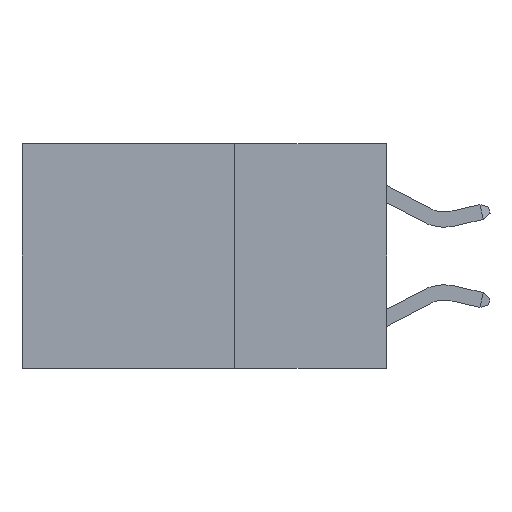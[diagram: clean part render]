
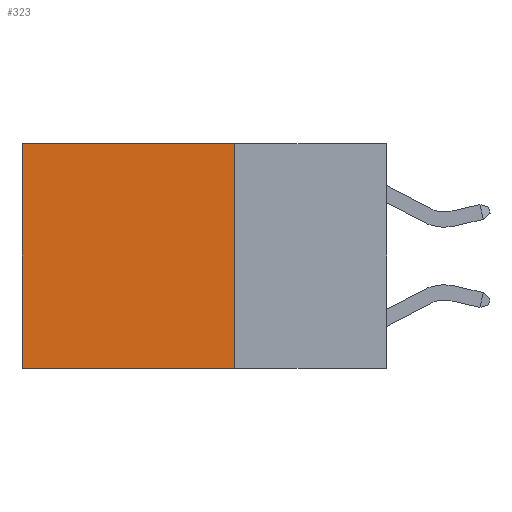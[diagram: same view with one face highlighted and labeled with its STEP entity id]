
A CAD part, left-side view. The second image highlights one B-rep face of the part: STEP entity #323.
In plain terms, the highlighted planar face has unit normal (-1, 0, 0).
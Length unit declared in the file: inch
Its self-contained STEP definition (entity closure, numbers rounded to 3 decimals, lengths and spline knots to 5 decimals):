
#47 = EDGE_CURVE ( 'NONE', #4395, #8776, #652, .T. ) ;
#245 = DIRECTION ( 'NONE',  ( 0., 1., 0. ) ) ;
#276 = VECTOR ( 'NONE', #245, 39.37008 ) ;
#323 = ADVANCED_FACE ( 'NONE', ( #2321 ), #8153, .F. ) ;
#652 = LINE ( 'NONE', #1391, #6294 ) ;
#1089 = VERTEX_POINT ( 'NONE', #1282 ) ;
#1282 = CARTESIAN_POINT ( 'NONE',  ( 0.2625, 0.6, 0. ) ) ;
#1391 = CARTESIAN_POINT ( 'NONE',  ( 0.2625, 0.25, 0. ) ) ;
#1537 = ORIENTED_EDGE ( 'NONE', *, *, #47, .F. ) ;
#1599 = CARTESIAN_POINT ( 'NONE',  ( 0.2625, 0.25, 0. ) ) ;
#1648 = EDGE_CURVE ( 'NONE', #8776, #8783, #3043, .T. ) ;
#1809 = CARTESIAN_POINT ( 'NONE',  ( 0.2625, 0.25, 0. ) ) ;
#2150 = LINE ( 'NONE', #5111, #7468 ) ;
#2187 = ORIENTED_EDGE ( 'NONE', *, *, #1648, .F. ) ;
#2321 = FACE_OUTER_BOUND ( 'NONE', #5531, .T. ) ;
#2572 = DIRECTION ( 'NONE',  ( 0., 0., -1. ) ) ;
#2839 = EDGE_CURVE ( 'NONE', #1089, #8783, #8261, .T. ) ;
#3043 = LINE ( 'NONE', #3908, #276 ) ;
#3132 = DIRECTION ( 'NONE',  ( 0., 1., 0. ) ) ;
#3908 = CARTESIAN_POINT ( 'NONE',  ( 0.2625, 0.25, -0.37 ) ) ;
#4324 = DIRECTION ( 'NONE',  ( 0., 0., -1. ) ) ;
#4357 = CARTESIAN_POINT ( 'NONE',  ( 0.2625, 0.25, -0.37 ) ) ;
#4395 = VERTEX_POINT ( 'NONE', #1809 ) ;
#5111 = CARTESIAN_POINT ( 'NONE',  ( 0.2625, 0.25, 0. ) ) ;
#5531 = EDGE_LOOP ( 'NONE', ( #7903, #2187, #1537, #7173 ) ) ;
#6037 = EDGE_CURVE ( 'NONE', #4395, #1089, #2150, .T. ) ;
#6179 = CARTESIAN_POINT ( 'NONE',  ( 0.2625, 0.6, 0. ) ) ;
#6294 = VECTOR ( 'NONE', #4324, 39.37008 ) ;
#6796 = DIRECTION ( 'NONE',  ( 1., 0., 0. ) ) ;
#6907 = AXIS2_PLACEMENT_3D ( 'NONE', #1599, #6796, #8248 ) ;
#7173 = ORIENTED_EDGE ( 'NONE', *, *, #6037, .T. ) ;
#7468 = VECTOR ( 'NONE', #3132, 39.37008 ) ;
#7878 = CARTESIAN_POINT ( 'NONE',  ( 0.2625, 0.6, -0.37 ) ) ;
#7903 = ORIENTED_EDGE ( 'NONE', *, *, #2839, .T. ) ;
#8153 = PLANE ( 'NONE',  #6907 ) ;
#8248 = DIRECTION ( 'NONE',  ( 0., 0., -1. ) ) ;
#8261 = LINE ( 'NONE', #6179, #8292 ) ;
#8292 = VECTOR ( 'NONE', #2572, 39.37008 ) ;
#8776 = VERTEX_POINT ( 'NONE', #4357 ) ;
#8783 = VERTEX_POINT ( 'NONE', #7878 ) ;
